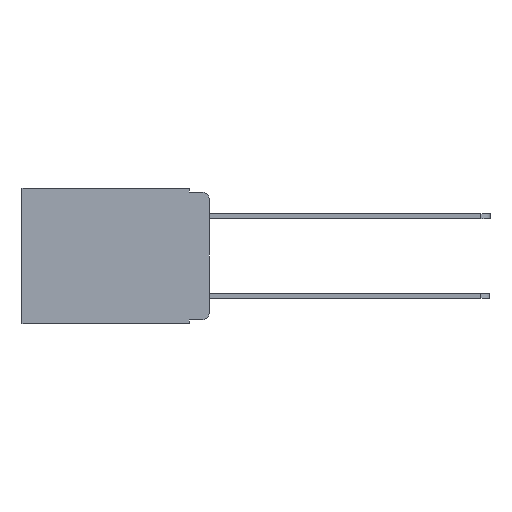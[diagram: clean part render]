
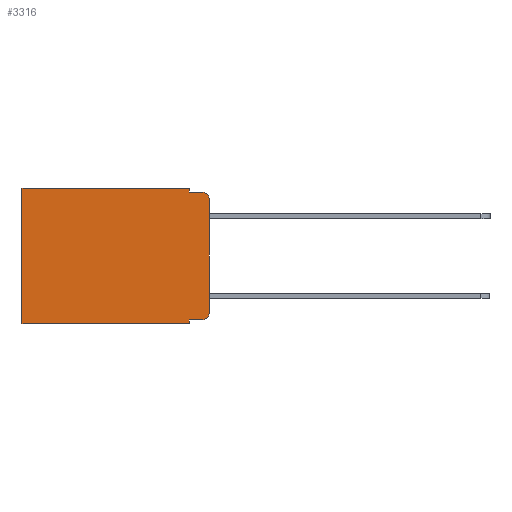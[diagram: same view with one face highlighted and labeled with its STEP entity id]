
A CAD part, left-side view. The second image highlights one B-rep face of the part: STEP entity #3316.
In plain terms, the highlighted planar face has unit normal (-1, 0, 0).
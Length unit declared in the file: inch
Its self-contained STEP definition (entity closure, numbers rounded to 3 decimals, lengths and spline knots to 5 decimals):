
#80 = DIRECTION ( 'NONE',  ( -1., 0., 0. ) ) ;
#285 = VECTOR ( 'NONE', #20000, 39.37008 ) ;
#1041 = CARTESIAN_POINT ( 'NONE',  ( 0.298, 0.051, 0. ) ) ;
#1273 = CARTESIAN_POINT ( 'NONE',  ( 0.298, 0.051, -0.01 ) ) ;
#1471 = VERTEX_POINT ( 'NONE', #22021 ) ;
#2226 = ORIENTED_EDGE ( 'NONE', *, *, #5600, .F. ) ;
#2242 = VECTOR ( 'NONE', #7764, 39.37008 ) ;
#2585 = DIRECTION ( 'NONE',  ( 0., 1., 0. ) ) ;
#2597 = DIRECTION ( 'NONE',  ( 0., 0., -1. ) ) ;
#3254 = CARTESIAN_POINT ( 'NONE',  ( 0.298, 0.051, 0. ) ) ;
#3263 = VERTEX_POINT ( 'NONE', #7109 ) ;
#3316 = ADVANCED_FACE ( 'NONE', ( #5121 ), #11696, .F. ) ;
#3369 = EDGE_CURVE ( 'NONE', #3444, #12329, #4036, .T. ) ;
#3444 = VERTEX_POINT ( 'NONE', #3254 ) ;
#4036 = LINE ( 'NONE', #10465, #21011 ) ;
#4218 = LINE ( 'NONE', #17814, #12283 ) ;
#4541 = EDGE_LOOP ( 'NONE', ( #13903, #7148, #15801, #5011, #14721, #14985, #5376, #2226, #19562, #9055 ) ) ;
#4552 = LINE ( 'NONE', #12875, #13724 ) ;
#4668 = VECTOR ( 'NONE', #2597, 39.37008 ) ;
#4786 = CARTESIAN_POINT ( 'NONE',  ( 0.298, 0., -0.313 ) ) ;
#4857 = DIRECTION ( 'NONE',  ( 0., 0., -1. ) ) ;
#4940 = LINE ( 'NONE', #1273, #285 ) ;
#5011 = ORIENTED_EDGE ( 'NONE', *, *, #3369, .F. ) ;
#5121 = FACE_OUTER_BOUND ( 'NONE', #4541, .T. ) ;
#5376 = ORIENTED_EDGE ( 'NONE', *, *, #20072, .F. ) ;
#5379 = LINE ( 'NONE', #6589, #13412 ) ;
#5600 = EDGE_CURVE ( 'NONE', #7269, #16915, #7225, .T. ) ;
#5809 = AXIS2_PLACEMENT_3D ( 'NONE', #14612, #11626, #11770 ) ;
#5883 = CARTESIAN_POINT ( 'NONE',  ( 0.298, 0.051, -0.333 ) ) ;
#6552 = CARTESIAN_POINT ( 'NONE',  ( 0.298, 0.051, -0.01 ) ) ;
#6589 = CARTESIAN_POINT ( 'NONE',  ( 0.298, 0., 0. ) ) ;
#7104 = AXIS2_PLACEMENT_3D ( 'NONE', #20082, #10002, #21715 ) ;
#7109 = CARTESIAN_POINT ( 'NONE',  ( 0.298, 0.02, -0.01 ) ) ;
#7148 = ORIENTED_EDGE ( 'NONE', *, *, #19191, .T. ) ;
#7225 = LINE ( 'NONE', #1041, #20167 ) ;
#7269 = VERTEX_POINT ( 'NONE', #5883 ) ;
#7322 = EDGE_CURVE ( 'NONE', #8934, #1471, #17288, .T. ) ;
#7376 = CIRCLE ( 'NONE', #12779, 0.02 ) ;
#7528 = EDGE_CURVE ( 'NONE', #12329, #3263, #4940, .T. ) ;
#7655 = DIRECTION ( 'NONE',  ( 0., 1., 0. ) ) ;
#7764 = DIRECTION ( 'NONE',  ( 0., -1., 0. ) ) ;
#8338 = CIRCLE ( 'NONE', #7104, 0.02 ) ;
#8934 = VERTEX_POINT ( 'NONE', #9569 ) ;
#9055 = ORIENTED_EDGE ( 'NONE', *, *, #17025, .T. ) ;
#9569 = CARTESIAN_POINT ( 'NONE',  ( 0.298, 0.473, 0. ) ) ;
#9709 = DIRECTION ( 'NONE',  ( 0., 0., -1. ) ) ;
#9793 = EDGE_CURVE ( 'NONE', #19685, #20998, #5379, .T. ) ;
#10002 = DIRECTION ( 'NONE',  ( -1., 0., 0. ) ) ;
#10465 = CARTESIAN_POINT ( 'NONE',  ( 0.298, 0.051, 0. ) ) ;
#10509 = CARTESIAN_POINT ( 'NONE',  ( 0.298, 0.02, -0.313 ) ) ;
#10891 = LINE ( 'NONE', #16292, #2242 ) ;
#11626 = DIRECTION ( 'NONE',  ( 1., 0., 0. ) ) ;
#11696 = PLANE ( 'NONE',  #5809 ) ;
#11770 = DIRECTION ( 'NONE',  ( 0., 0., -1. ) ) ;
#12184 = DIRECTION ( 'NONE',  ( 0., 0., -1. ) ) ;
#12283 = VECTOR ( 'NONE', #7655, 39.37008 ) ;
#12329 = VERTEX_POINT ( 'NONE', #6552 ) ;
#12779 = AXIS2_PLACEMENT_3D ( 'NONE', #10509, #80, #12184 ) ;
#12875 = CARTESIAN_POINT ( 'NONE',  ( 0.298, 0., 0. ) ) ;
#12887 = CARTESIAN_POINT ( 'NONE',  ( 0.298, 0.473, 0. ) ) ;
#13412 = VECTOR ( 'NONE', #20195, 39.37008 ) ;
#13724 = VECTOR ( 'NONE', #2585, 39.37008 ) ;
#13788 = CARTESIAN_POINT ( 'NONE',  ( 0.298, 0.02, -0.333 ) ) ;
#13903 = ORIENTED_EDGE ( 'NONE', *, *, #9793, .F. ) ;
#14612 = CARTESIAN_POINT ( 'NONE',  ( 0.298, 0., 0. ) ) ;
#14721 = ORIENTED_EDGE ( 'NONE', *, *, #18414, .T. ) ;
#14985 = ORIENTED_EDGE ( 'NONE', *, *, #7322, .T. ) ;
#15801 = ORIENTED_EDGE ( 'NONE', *, *, #7528, .F. ) ;
#16207 = EDGE_CURVE ( 'NONE', #7269, #18760, #10891, .T. ) ;
#16292 = CARTESIAN_POINT ( 'NONE',  ( 0.298, 0.051, -0.333 ) ) ;
#16915 = VERTEX_POINT ( 'NONE', #21832 ) ;
#17025 = EDGE_CURVE ( 'NONE', #18760, #20998, #7376, .T. ) ;
#17288 = LINE ( 'NONE', #12887, #4668 ) ;
#17814 = CARTESIAN_POINT ( 'NONE',  ( 0.298, 0., -0.343 ) ) ;
#18414 = EDGE_CURVE ( 'NONE', #3444, #8934, #4552, .T. ) ;
#18760 = VERTEX_POINT ( 'NONE', #13788 ) ;
#19191 = EDGE_CURVE ( 'NONE', #19685, #3263, #8338, .T. ) ;
#19562 = ORIENTED_EDGE ( 'NONE', *, *, #16207, .T. ) ;
#19640 = CARTESIAN_POINT ( 'NONE',  ( 0.298, 0., -0.03 ) ) ;
#19685 = VERTEX_POINT ( 'NONE', #19640 ) ;
#20000 = DIRECTION ( 'NONE',  ( 0., -1., 0. ) ) ;
#20072 = EDGE_CURVE ( 'NONE', #16915, #1471, #4218, .T. ) ;
#20082 = CARTESIAN_POINT ( 'NONE',  ( 0.298, 0.02, -0.03 ) ) ;
#20167 = VECTOR ( 'NONE', #9709, 39.37008 ) ;
#20195 = DIRECTION ( 'NONE',  ( 0., 0., -1. ) ) ;
#20998 = VERTEX_POINT ( 'NONE', #4786 ) ;
#21011 = VECTOR ( 'NONE', #4857, 39.37008 ) ;
#21715 = DIRECTION ( 'NONE',  ( 0., 0., -1. ) ) ;
#21832 = CARTESIAN_POINT ( 'NONE',  ( 0.298, 0.051, -0.343 ) ) ;
#22021 = CARTESIAN_POINT ( 'NONE',  ( 0.298, 0.473, -0.343 ) ) ;
